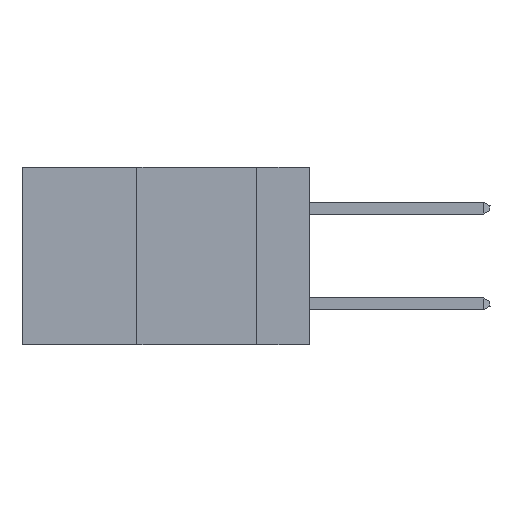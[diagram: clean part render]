
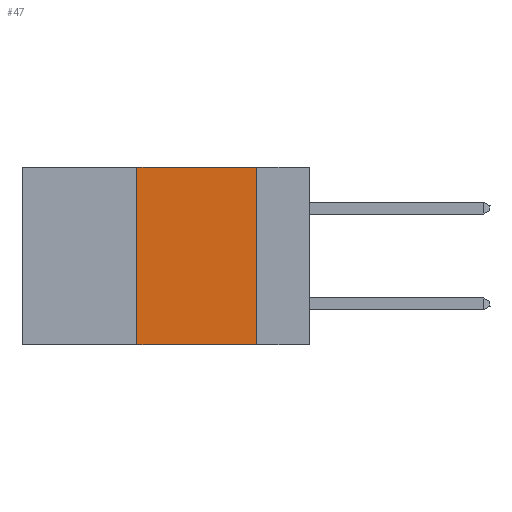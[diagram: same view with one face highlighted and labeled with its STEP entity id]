
A CAD part, left-side view. The second image highlights one B-rep face of the part: STEP entity #47.
In plain terms, the highlighted planar face has unit normal (-1, 0, 0).
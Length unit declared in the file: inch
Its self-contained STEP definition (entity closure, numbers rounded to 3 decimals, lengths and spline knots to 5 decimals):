
#47 = ADVANCED_FACE ( 'NONE', ( #19726 ), #4486, .F. ) ;
#1492 = VERTEX_POINT ( 'NONE', #13677 ) ;
#1783 = CARTESIAN_POINT ( 'NONE',  ( 0., 0.6, -0.37 ) ) ;
#2445 = ORIENTED_EDGE ( 'NONE', *, *, #23323, .T. ) ;
#4486 = PLANE ( 'NONE',  #17115 ) ;
#6356 = DIRECTION ( 'NONE',  ( 0., 0., -1. ) ) ;
#6570 = VECTOR ( 'NONE', #12833, 39.37008 ) ;
#6803 = DIRECTION ( 'NONE',  ( 0., 0., 1. ) ) ;
#7618 = LINE ( 'NONE', #22320, #16876 ) ;
#8593 = EDGE_CURVE ( 'NONE', #20760, #9534, #10598, .T. ) ;
#9421 = DIRECTION ( 'NONE',  ( 0., -1., 0. ) ) ;
#9534 = VERTEX_POINT ( 'NONE', #10637 ) ;
#10039 = VECTOR ( 'NONE', #6803, 39.37008 ) ;
#10598 = LINE ( 'NONE', #12280, #10039 ) ;
#10637 = CARTESIAN_POINT ( 'NONE',  ( 0., 0.36, 0. ) ) ;
#11033 = DIRECTION ( 'NONE',  ( 0., 0., -1. ) ) ;
#12032 = LINE ( 'NONE', #1783, #6570 ) ;
#12280 = CARTESIAN_POINT ( 'NONE',  ( 0., 0.36, 0. ) ) ;
#12455 = LINE ( 'NONE', #18421, #21702 ) ;
#12833 = DIRECTION ( 'NONE',  ( 0., -1., 0. ) ) ;
#13243 = EDGE_LOOP ( 'NONE', ( #14241, #15428, #20950, #2445 ) ) ;
#13677 = CARTESIAN_POINT ( 'NONE',  ( 0., 0.11, 0. ) ) ;
#14241 = ORIENTED_EDGE ( 'NONE', *, *, #18048, .F. ) ;
#15428 = ORIENTED_EDGE ( 'NONE', *, *, #16724, .F. ) ;
#15534 = CARTESIAN_POINT ( 'NONE',  ( 0., 0.6, 0. ) ) ;
#15709 = CARTESIAN_POINT ( 'NONE',  ( 0., 0.36, -0.37 ) ) ;
#16724 = EDGE_CURVE ( 'NONE', #9534, #1492, #7618, .T. ) ;
#16876 = VECTOR ( 'NONE', #9421, 39.37008 ) ;
#17115 = AXIS2_PLACEMENT_3D ( 'NONE', #15534, #17418, #6356 ) ;
#17418 = DIRECTION ( 'NONE',  ( 1., 0., 0. ) ) ;
#18048 = EDGE_CURVE ( 'NONE', #1492, #22109, #12455, .T. ) ;
#18421 = CARTESIAN_POINT ( 'NONE',  ( 0., 0.11, 0. ) ) ;
#18610 = CARTESIAN_POINT ( 'NONE',  ( 0., 0.11, -0.37 ) ) ;
#19726 = FACE_OUTER_BOUND ( 'NONE', #13243, .T. ) ;
#20760 = VERTEX_POINT ( 'NONE', #15709 ) ;
#20950 = ORIENTED_EDGE ( 'NONE', *, *, #8593, .F. ) ;
#21702 = VECTOR ( 'NONE', #11033, 39.37008 ) ;
#22109 = VERTEX_POINT ( 'NONE', #18610 ) ;
#22320 = CARTESIAN_POINT ( 'NONE',  ( 0., 0.6, 0. ) ) ;
#23323 = EDGE_CURVE ( 'NONE', #20760, #22109, #12032, .T. ) ;
